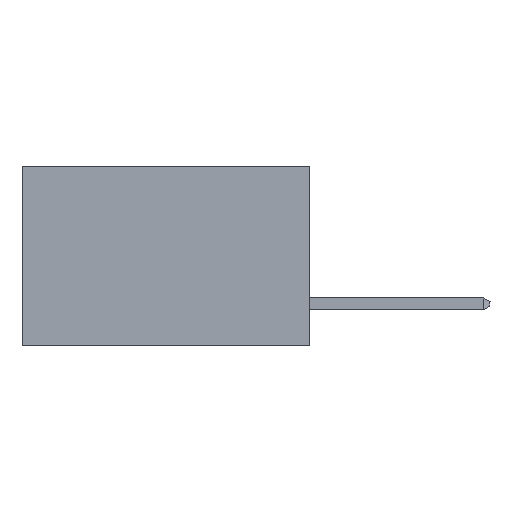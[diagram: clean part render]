
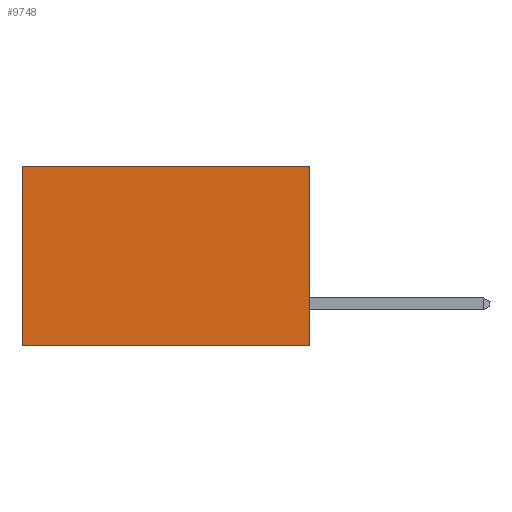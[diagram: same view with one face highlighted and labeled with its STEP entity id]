
A CAD part, left-side view. The second image highlights one B-rep face of the part: STEP entity #9748.
In plain terms, the highlighted planar face has unit normal (-1, 0, 0).
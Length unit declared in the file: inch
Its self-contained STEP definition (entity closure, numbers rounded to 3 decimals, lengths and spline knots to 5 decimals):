
#2649 = VERTEX_POINT ( 'NONE', #10853 ) ;
#3094 = LINE ( 'NONE', #9076, #7208 ) ;
#3495 = DIRECTION ( 'NONE',  ( 1., 0., 0. ) ) ;
#3626 = EDGE_CURVE ( 'NONE', #6738, #14518, #3094, .T. ) ;
#4287 = VECTOR ( 'NONE', #7311, 39.37008 ) ;
#4441 = EDGE_CURVE ( 'NONE', #8186, #6738, #9049, .T. ) ;
#4523 = CARTESIAN_POINT ( 'NONE',  ( 0.2875, 0., 0. ) ) ;
#4724 = ORIENTED_EDGE ( 'NONE', *, *, #5684, .T. ) ;
#4992 = VECTOR ( 'NONE', #11443, 39.37008 ) ;
#4996 = DIRECTION ( 'NONE',  ( 0., 0., -1. ) ) ;
#5122 = AXIS2_PLACEMENT_3D ( 'NONE', #6441, #3495, #4996 ) ;
#5375 = DIRECTION ( 'NONE',  ( 0., 0., -1. ) ) ;
#5684 = EDGE_CURVE ( 'NONE', #8186, #2649, #12218, .T. ) ;
#6119 = CARTESIAN_POINT ( 'NONE',  ( 0.2875, 0., -0.375 ) ) ;
#6441 = CARTESIAN_POINT ( 'NONE',  ( 0.2875, 0., -0.375 ) ) ;
#6738 = VERTEX_POINT ( 'NONE', #15807 ) ;
#7208 = VECTOR ( 'NONE', #7740, 39.37008 ) ;
#7218 = PLANE ( 'NONE',  #5122 ) ;
#7311 = DIRECTION ( 'NONE',  ( 0., 1., 0. ) ) ;
#7346 = FACE_OUTER_BOUND ( 'NONE', #13069, .T. ) ;
#7740 = DIRECTION ( 'NONE',  ( 0., 1., 0. ) ) ;
#8074 = CARTESIAN_POINT ( 'NONE',  ( 0.2875, 0.6, -0.375 ) ) ;
#8186 = VERTEX_POINT ( 'NONE', #17575 ) ;
#8636 = ORIENTED_EDGE ( 'NONE', *, *, #16650, .T. ) ;
#9004 = ORIENTED_EDGE ( 'NONE', *, *, #3626, .F. ) ;
#9049 = LINE ( 'NONE', #6119, #4992 ) ;
#9076 = CARTESIAN_POINT ( 'NONE',  ( 0.2875, 0., -0.375 ) ) ;
#9748 = ADVANCED_FACE ( 'NONE', ( #7346 ), #7218, .F. ) ;
#10853 = CARTESIAN_POINT ( 'NONE',  ( 0.2875, 0.6, 0. ) ) ;
#11088 = CARTESIAN_POINT ( 'NONE',  ( 0.2875, 0.6, -0.375 ) ) ;
#11210 = VECTOR ( 'NONE', #5375, 39.37008 ) ;
#11443 = DIRECTION ( 'NONE',  ( 0., 0., -1. ) ) ;
#12218 = LINE ( 'NONE', #4523, #4287 ) ;
#13069 = EDGE_LOOP ( 'NONE', ( #8636, #9004, #16923, #4724 ) ) ;
#14518 = VERTEX_POINT ( 'NONE', #11088 ) ;
#15807 = CARTESIAN_POINT ( 'NONE',  ( 0.2875, 0., -0.375 ) ) ;
#16545 = LINE ( 'NONE', #8074, #11210 ) ;
#16650 = EDGE_CURVE ( 'NONE', #2649, #14518, #16545, .T. ) ;
#16923 = ORIENTED_EDGE ( 'NONE', *, *, #4441, .F. ) ;
#17575 = CARTESIAN_POINT ( 'NONE',  ( 0.2875, 0., 0. ) ) ;
